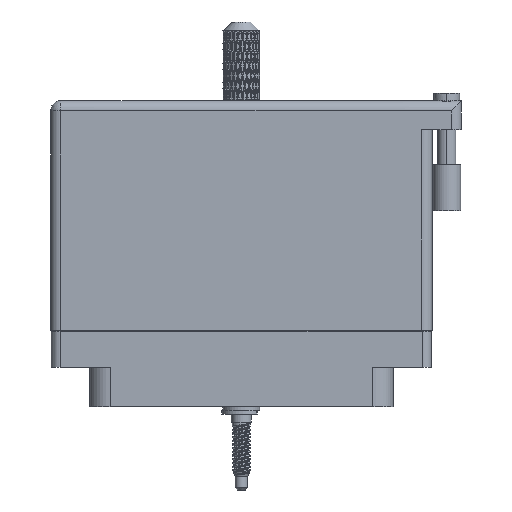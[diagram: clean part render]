
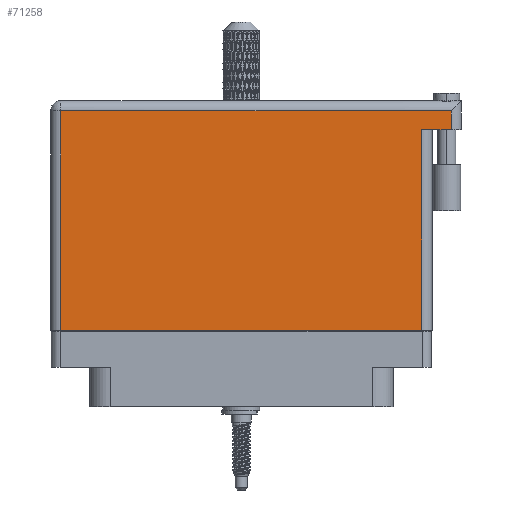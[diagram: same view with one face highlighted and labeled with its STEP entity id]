
A CAD part, front view. The second image highlights one B-rep face of the part: STEP entity #71258.
In plain terms, the highlighted face is planar.
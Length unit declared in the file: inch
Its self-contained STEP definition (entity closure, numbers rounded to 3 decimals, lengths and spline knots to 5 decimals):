
#2292 = CARTESIAN_POINT ( 'NONE',  ( -1.23, -0.1, 0.4495 ) ) ;
#3123 = EDGE_CURVE ( 'NONE', #101312, #5001, #21032, .T. ) ;
#5001 = VERTEX_POINT ( 'NONE', #2292 ) ;
#5229 = CARTESIAN_POINT ( 'NONE',  ( 1.5, 1.269, 0.4495 ) ) ;
#6212 = FACE_OUTER_BOUND ( 'NONE', #83950, .T. ) ;
#6367 = CARTESIAN_POINT ( 'NONE',  ( 1.43, 1.269, 0.4495 ) ) ;
#10052 = CARTESIAN_POINT ( 'NONE',  ( -1.3, 1.466, 0.4495 ) ) ;
#10450 = DIRECTION ( 'NONE',  ( -1., 0., 0. ) ) ;
#13520 = VERTEX_POINT ( 'NONE', #109580 ) ;
#20311 = ORIENTED_EDGE ( 'NONE', *, *, #54020, .F. ) ;
#20784 = VERTEX_POINT ( 'NONE', #6367 ) ;
#21032 = LINE ( 'NONE', #31062, #86211 ) ;
#22482 = DIRECTION ( 'NONE',  ( 0., 1., 0. ) ) ;
#24219 = VECTOR ( 'NONE', #49087, 39.37008 ) ;
#24561 = EDGE_CURVE ( 'NONE', #37443, #100961, #103696, .T. ) ;
#26946 = CARTESIAN_POINT ( 'NONE',  ( 1.23, -0.1, 0.4495 ) ) ;
#29809 = DIRECTION ( 'NONE',  ( 0., 1., 0. ) ) ;
#31062 = CARTESIAN_POINT ( 'NONE',  ( -1.23, -0.1, 0.4495 ) ) ;
#36731 = VECTOR ( 'NONE', #73472, 39.37008 ) ;
#37443 = VERTEX_POINT ( 'NONE', #26946 ) ;
#38950 = ORIENTED_EDGE ( 'NONE', *, *, #72189, .T. ) ;
#44881 = DIRECTION ( 'NONE',  ( 0., 0., -1. ) ) ;
#45223 = CARTESIAN_POINT ( 'NONE',  ( -1.23, 1.396, 0.4495 ) ) ;
#46506 = CARTESIAN_POINT ( 'NONE',  ( -1.3, 1.396, 0.4495 ) ) ;
#48267 = LINE ( 'NONE', #103313, #24219 ) ;
#49087 = DIRECTION ( 'NONE',  ( 1., 0., 0. ) ) ;
#52086 = AXIS2_PLACEMENT_3D ( 'NONE', #10052, #44881, #10450 ) ;
#54020 = EDGE_CURVE ( 'NONE', #20784, #100961, #104035, .T. ) ;
#60328 = ORIENTED_EDGE ( 'NONE', *, *, #3123, .T. ) ;
#68728 = DIRECTION ( 'NONE',  ( 0., -1., 0. ) ) ;
#69462 = CARTESIAN_POINT ( 'NONE',  ( 1.43, 1.466, 0.4495 ) ) ;
#70644 = LINE ( 'NONE', #69462, #115984 ) ;
#71258 = ADVANCED_FACE ( 'NONE', ( #6212 ), #82146, .F. ) ;
#72189 = EDGE_CURVE ( 'NONE', #13520, #101312, #78026, .T. ) ;
#73472 = DIRECTION ( 'NONE',  ( -1., 0., 0. ) ) ;
#75587 = VECTOR ( 'NONE', #22482, 39.37008 ) ;
#78026 = LINE ( 'NONE', #46506, #36731 ) ;
#82146 = PLANE ( 'NONE',  #52086 ) ;
#83950 = EDGE_LOOP ( 'NONE', ( #92644, #115403, #20311, #91219, #38950, #60328 ) ) ;
#86211 = VECTOR ( 'NONE', #68728, 39.37008 ) ;
#90207 = EDGE_CURVE ( 'NONE', #20784, #13520, #70644, .T. ) ;
#91219 = ORIENTED_EDGE ( 'NONE', *, *, #90207, .T. ) ;
#92644 = ORIENTED_EDGE ( 'NONE', *, *, #115555, .T. ) ;
#93676 = CARTESIAN_POINT ( 'NONE',  ( 1.23, 1.269, 0.4495 ) ) ;
#96225 = DIRECTION ( 'NONE',  ( -1., 0., 0. ) ) ;
#100961 = VERTEX_POINT ( 'NONE', #93676 ) ;
#101312 = VERTEX_POINT ( 'NONE', #45223 ) ;
#103313 = CARTESIAN_POINT ( 'NONE',  ( -1.3, -0.1, 0.4495 ) ) ;
#103696 = LINE ( 'NONE', #113523, #75587 ) ;
#104035 = LINE ( 'NONE', #5229, #109802 ) ;
#109580 = CARTESIAN_POINT ( 'NONE',  ( 1.43, 1.396, 0.4495 ) ) ;
#109802 = VECTOR ( 'NONE', #96225, 39.37008 ) ;
#113523 = CARTESIAN_POINT ( 'NONE',  ( 1.23, 1.269, 0.4495 ) ) ;
#115403 = ORIENTED_EDGE ( 'NONE', *, *, #24561, .T. ) ;
#115555 = EDGE_CURVE ( 'NONE', #5001, #37443, #48267, .T. ) ;
#115984 = VECTOR ( 'NONE', #29809, 39.37008 ) ;
